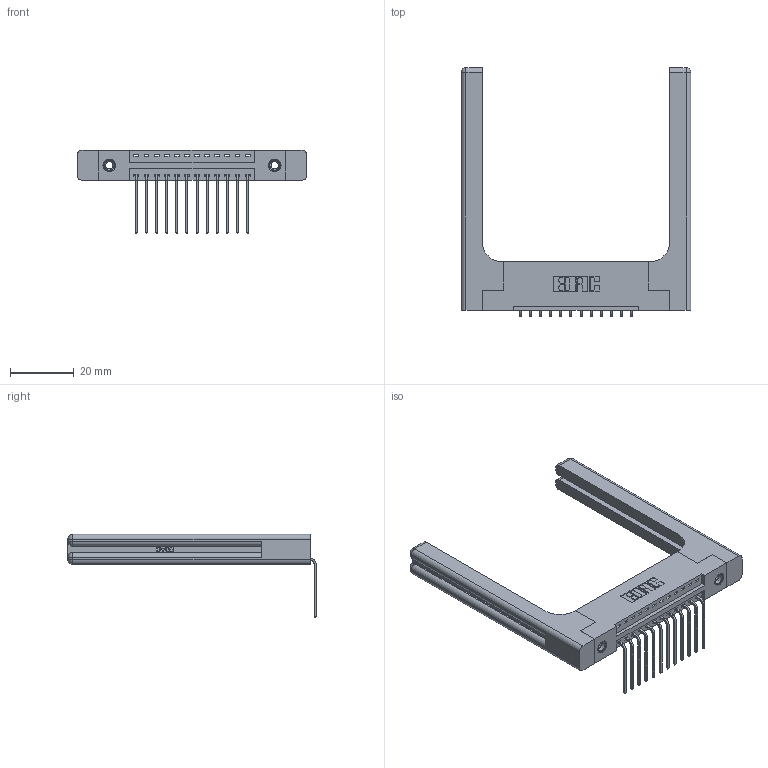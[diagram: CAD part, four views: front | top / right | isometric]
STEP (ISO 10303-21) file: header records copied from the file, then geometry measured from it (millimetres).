
FILE_DESCRIPTION (( 'STEP AP203' ), '1' );
FILE_NAME ('396-012-559-158.STEP', '2019-10-31T20:19:44', ( '' ), ( '' ), 'SwSTEP 2.0', 'SolidWorks 2016', '' );
FILE_SCHEMA (( 'CONFIG_CONTROL_DESIGN' ));
Length unit declared in the file: inch
Products named in the file (5): 346 Part_Flush Mounting Lugs - 0.156 Dia-TH; 345-292-001_558 559 Tail - 1; 345-250-001_345-250-001-102; 346-220-058_345-220-058; 396-012-559-158
Assembly tree (17 placements, depth 2):
  396-012-559-158
    346 Part_Flush Mounting Lugs - 0.156 Dia-TH
    345-292-001_558 559 Tail - 1  x12
    345-250-001_345-250-001-102  x2
    346-220-058_345-220-058  x2
Bounding box: 72.16 x 78.04 x 26.16 mm (x, y, z)
Volume: 14259.1 mm3; surface area: 13509.4 mm2
Topology: 17 solids, 17 shells, 1098 faces, 3179 edges, 2082 vertices
Faces by surface type: plane 728, cylinder 310, bspline 36, cone 12, sphere 8, torus 4
Entity records: 16752 total; most frequent: CARTESIAN_POINT 3861, ORIENTED_EDGE 2604, DIRECTION 2374, EDGE_CURVE 1302, VECTOR 1030, LINE 1030, VERTEX_POINT 858, AXIS2_PLACEMENT_3D 672
